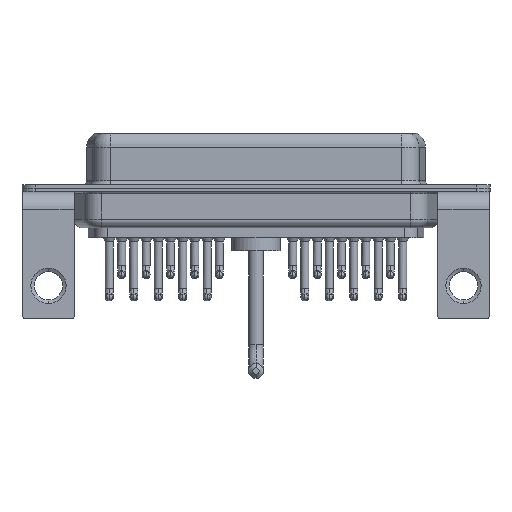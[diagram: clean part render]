
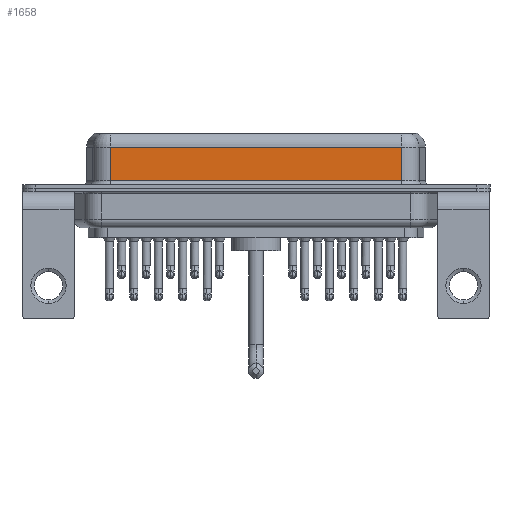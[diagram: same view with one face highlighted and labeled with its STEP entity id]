
A CAD part, front view. The second image highlights one B-rep face of the part: STEP entity #1658.
In plain terms, the highlighted planar face has unit normal (0, -1, 0).
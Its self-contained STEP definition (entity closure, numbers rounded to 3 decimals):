
#173 = ORIENTED_EDGE ( 'NONE', *, *, #4874, .T. ) ;
#501 = FACE_OUTER_BOUND ( 'NONE', #13160, .T. ) ;
#900 = CARTESIAN_POINT ( 'NONE',  ( 7.013, -3.95, 0.9 ) ) ;
#1658 = ADVANCED_FACE ( 'NONE', ( #501 ), #7237, .F. ) ;
#2574 = DIRECTION ( 'NONE',  ( 1., 0., 0. ) ) ;
#3482 = AXIS2_PLACEMENT_3D ( 'NONE', #7720, #14978, #4157 ) ;
#4157 = DIRECTION ( 'NONE',  ( 0., 0., 1. ) ) ;
#4874 = EDGE_CURVE ( 'NONE', #14594, #21000, #15197, .T. ) ;
#6219 = CARTESIAN_POINT ( 'NONE',  ( 40.037, -3.95, 4.65 ) ) ;
#6559 = EDGE_CURVE ( 'NONE', #23418, #13923, #21913, .T. ) ;
#7237 = PLANE ( 'NONE',  #3482 ) ;
#7720 = CARTESIAN_POINT ( 'NONE',  ( 40.037, -3.95, 6.4 ) ) ;
#7804 = CARTESIAN_POINT ( 'NONE',  ( 7.013, -3.95, 4.65 ) ) ;
#8235 = LINE ( 'NONE', #15487, #14870 ) ;
#9624 = CARTESIAN_POINT ( 'NONE',  ( 7.013, -3.95, 6.4 ) ) ;
#10899 = EDGE_CURVE ( 'NONE', #21000, #13923, #8235, .T. ) ;
#11010 = ORIENTED_EDGE ( 'NONE', *, *, #6559, .F. ) ;
#11526 = DIRECTION ( 'NONE',  ( 0., 0., -1. ) ) ;
#11673 = VECTOR ( 'NONE', #16352, 1000. ) ;
#12576 = EDGE_CURVE ( 'NONE', #23418, #14594, #15685, .T. ) ;
#13160 = EDGE_LOOP ( 'NONE', ( #11010, #14739, #173, #16130 ) ) ;
#13429 = VECTOR ( 'NONE', #11526, 1000. ) ;
#13896 = DIRECTION ( 'NONE',  ( -1., 0., 0. ) ) ;
#13923 = VERTEX_POINT ( 'NONE', #20290 ) ;
#14594 = VERTEX_POINT ( 'NONE', #7804 ) ;
#14739 = ORIENTED_EDGE ( 'NONE', *, *, #12576, .T. ) ;
#14870 = VECTOR ( 'NONE', #2574, 1000. ) ;
#14978 = DIRECTION ( 'NONE',  ( 0., 1., 0. ) ) ;
#15197 = LINE ( 'NONE', #9624, #13429 ) ;
#15487 = CARTESIAN_POINT ( 'NONE',  ( 40.037, -3.95, 0.9 ) ) ;
#15685 = LINE ( 'NONE', #22893, #20750 ) ;
#16130 = ORIENTED_EDGE ( 'NONE', *, *, #10899, .T. ) ;
#16352 = DIRECTION ( 'NONE',  ( 0., 0., -1. ) ) ;
#20290 = CARTESIAN_POINT ( 'NONE',  ( 40.037, -3.95, 0.9 ) ) ;
#20750 = VECTOR ( 'NONE', #13896, 1000. ) ;
#21000 = VERTEX_POINT ( 'NONE', #900 ) ;
#21563 = CARTESIAN_POINT ( 'NONE',  ( 40.037, -3.95, 6.4 ) ) ;
#21913 = LINE ( 'NONE', #21563, #11673 ) ;
#22893 = CARTESIAN_POINT ( 'NONE',  ( 40.037, -3.95, 4.65 ) ) ;
#23418 = VERTEX_POINT ( 'NONE', #6219 ) ;
